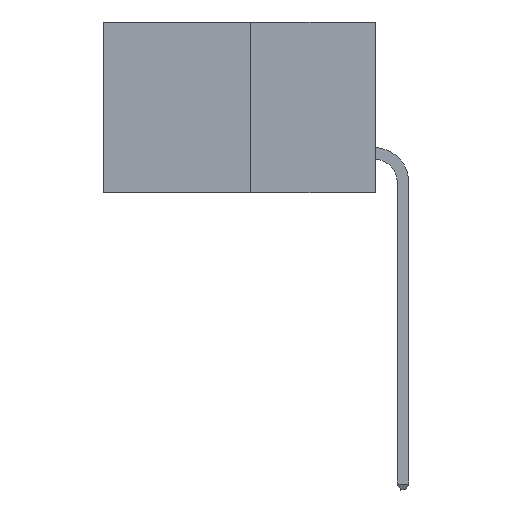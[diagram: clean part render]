
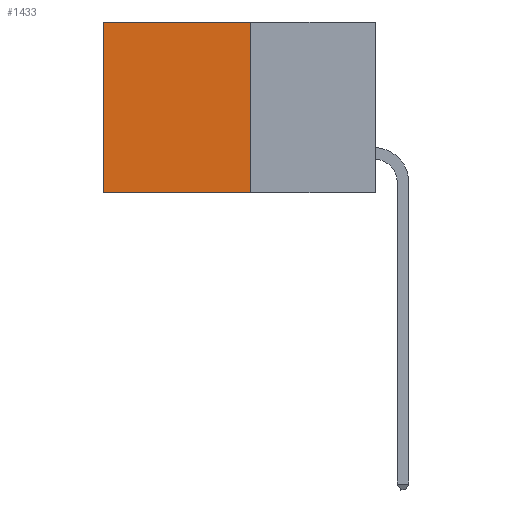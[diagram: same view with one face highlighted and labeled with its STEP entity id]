
A CAD part, left-side view. The second image highlights one B-rep face of the part: STEP entity #1433.
In plain terms, the highlighted planar face has unit normal (-1, 0, 0).
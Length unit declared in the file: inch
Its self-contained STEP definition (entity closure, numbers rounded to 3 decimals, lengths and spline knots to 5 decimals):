
#1433 = ADVANCED_FACE ( 'NONE', ( #10453 ), #12309, .F. ) ;
#1671 = CARTESIAN_POINT ( 'NONE',  ( 0.277, 0.27, -0.37 ) ) ;
#1758 = CARTESIAN_POINT ( 'NONE',  ( 0.277, 0.59, -0.37 ) ) ;
#2517 = VECTOR ( 'NONE', #10448, 39.37008 ) ;
#2800 = VERTEX_POINT ( 'NONE', #13388 ) ;
#2843 = VERTEX_POINT ( 'NONE', #13996 ) ;
#2862 = ORIENTED_EDGE ( 'NONE', *, *, #13495, .F. ) ;
#2891 = DIRECTION ( 'NONE',  ( 0., 1., 0. ) ) ;
#2981 = DIRECTION ( 'NONE',  ( 0., 0., -1. ) ) ;
#3188 = CARTESIAN_POINT ( 'NONE',  ( 0.277, 0.59, 0. ) ) ;
#3249 = ORIENTED_EDGE ( 'NONE', *, *, #6313, .F. ) ;
#3838 = VECTOR ( 'NONE', #12644, 39.37008 ) ;
#3983 = CARTESIAN_POINT ( 'NONE',  ( 0.277, 0.27, -0.37 ) ) ;
#4285 = VECTOR ( 'NONE', #2981, 39.37008 ) ;
#6131 = VERTEX_POINT ( 'NONE', #3983 ) ;
#6313 = EDGE_CURVE ( 'NONE', #2800, #6131, #9407, .T. ) ;
#6337 = EDGE_LOOP ( 'NONE', ( #15463, #2862, #3249, #6505 ) ) ;
#6505 = ORIENTED_EDGE ( 'NONE', *, *, #6896, .T. ) ;
#6896 = EDGE_CURVE ( 'NONE', #2800, #14411, #10337, .T. ) ;
#7919 = LINE ( 'NONE', #1758, #4285 ) ;
#9407 = LINE ( 'NONE', #15237, #2517 ) ;
#9703 = AXIS2_PLACEMENT_3D ( 'NONE', #13620, #13746, #14884 ) ;
#10337 = LINE ( 'NONE', #11418, #3838 ) ;
#10448 = DIRECTION ( 'NONE',  ( 0., 0., -1. ) ) ;
#10453 = FACE_OUTER_BOUND ( 'NONE', #6337, .T. ) ;
#10967 = EDGE_CURVE ( 'NONE', #14411, #2843, #7919, .T. ) ;
#11245 = VECTOR ( 'NONE', #2891, 39.37008 ) ;
#11418 = CARTESIAN_POINT ( 'NONE',  ( 0.277, 0.27, 0. ) ) ;
#11634 = LINE ( 'NONE', #1671, #11245 ) ;
#12309 = PLANE ( 'NONE',  #9703 ) ;
#12644 = DIRECTION ( 'NONE',  ( 0., 1., 0. ) ) ;
#13388 = CARTESIAN_POINT ( 'NONE',  ( 0.277, 0.27, 0. ) ) ;
#13495 = EDGE_CURVE ( 'NONE', #6131, #2843, #11634, .T. ) ;
#13620 = CARTESIAN_POINT ( 'NONE',  ( 0.277, 0.27, -0.37 ) ) ;
#13746 = DIRECTION ( 'NONE',  ( 1., 0., 0. ) ) ;
#13996 = CARTESIAN_POINT ( 'NONE',  ( 0.277, 0.59, -0.37 ) ) ;
#14411 = VERTEX_POINT ( 'NONE', #3188 ) ;
#14884 = DIRECTION ( 'NONE',  ( 0., 0., -1. ) ) ;
#15237 = CARTESIAN_POINT ( 'NONE',  ( 0.277, 0.27, -0.37 ) ) ;
#15463 = ORIENTED_EDGE ( 'NONE', *, *, #10967, .T. ) ;
